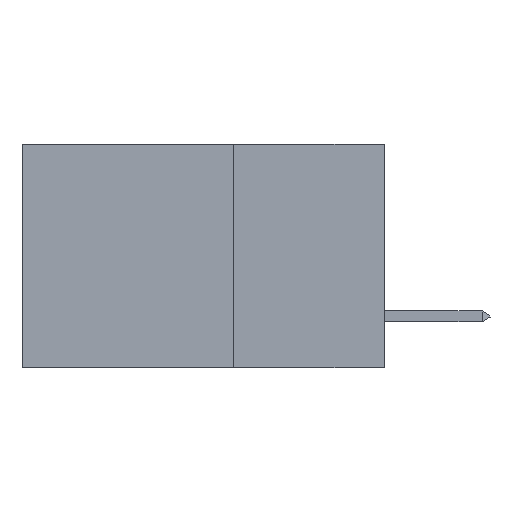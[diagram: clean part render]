
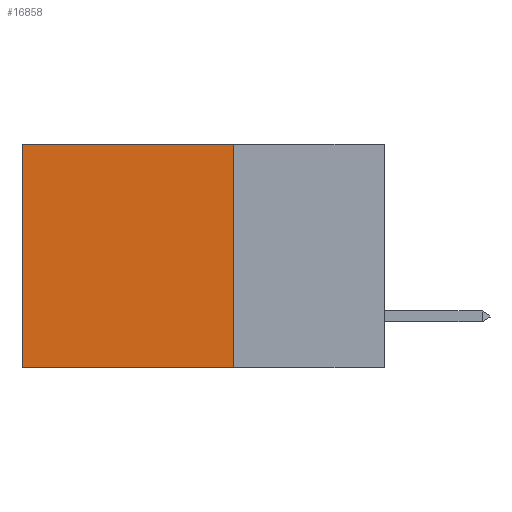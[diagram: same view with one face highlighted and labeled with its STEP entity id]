
A CAD part, left-side view. The second image highlights one B-rep face of the part: STEP entity #16858.
In plain terms, the highlighted planar face has unit normal (-1, 0, 0).
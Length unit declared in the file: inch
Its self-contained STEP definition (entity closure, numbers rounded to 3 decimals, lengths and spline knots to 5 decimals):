
#8 = DIRECTION ( 'NONE',  ( 0., 0., -1. ) ) ;
#34 = VERTEX_POINT ( 'NONE', #1742 ) ;
#244 = EDGE_LOOP ( 'NONE', ( #3949, #446, #4889, #4428 ) ) ;
#373 = CARTESIAN_POINT ( 'NONE',  ( 0.2875, 0.25, 0. ) ) ;
#446 = ORIENTED_EDGE ( 'NONE', *, *, #16270, .F. ) ;
#865 = VERTEX_POINT ( 'NONE', #12665 ) ;
#951 = EDGE_CURVE ( 'NONE', #34, #3635, #13948, .T. ) ;
#1742 = CARTESIAN_POINT ( 'NONE',  ( 0.2875, 0.6, 0. ) ) ;
#2558 = VERTEX_POINT ( 'NONE', #16355 ) ;
#2564 = CARTESIAN_POINT ( 'NONE',  ( 0.2875, 0.25, -0.37 ) ) ;
#3086 = CARTESIAN_POINT ( 'NONE',  ( 0.2875, 0.6, -0.37 ) ) ;
#3614 = FACE_OUTER_BOUND ( 'NONE', #244, .T. ) ;
#3635 = VERTEX_POINT ( 'NONE', #3086 ) ;
#3949 = ORIENTED_EDGE ( 'NONE', *, *, #951, .T. ) ;
#3950 = DIRECTION ( 'NONE',  ( 0., 1., 0. ) ) ;
#4428 = ORIENTED_EDGE ( 'NONE', *, *, #7048, .T. ) ;
#4889 = ORIENTED_EDGE ( 'NONE', *, *, #8742, .F. ) ;
#6504 = CARTESIAN_POINT ( 'NONE',  ( 0.2875, 0.25, 0. ) ) ;
#6998 = LINE ( 'NONE', #373, #10014 ) ;
#7048 = EDGE_CURVE ( 'NONE', #2558, #34, #6998, .T. ) ;
#7086 = DIRECTION ( 'NONE',  ( 0., 1., 0. ) ) ;
#7163 = VECTOR ( 'NONE', #8, 39.37008 ) ;
#7591 = VECTOR ( 'NONE', #12647, 39.37008 ) ;
#7809 = DIRECTION ( 'NONE',  ( 0., 0., -1. ) ) ;
#7985 = LINE ( 'NONE', #10564, #7163 ) ;
#8742 = EDGE_CURVE ( 'NONE', #2558, #865, #7985, .T. ) ;
#9997 = LINE ( 'NONE', #2564, #16313 ) ;
#10014 = VECTOR ( 'NONE', #7086, 39.37008 ) ;
#10540 = AXIS2_PLACEMENT_3D ( 'NONE', #6504, #15398, #7809 ) ;
#10564 = CARTESIAN_POINT ( 'NONE',  ( 0.2875, 0.25, 0. ) ) ;
#12647 = DIRECTION ( 'NONE',  ( 0., 0., -1. ) ) ;
#12665 = CARTESIAN_POINT ( 'NONE',  ( 0.2875, 0.25, -0.37 ) ) ;
#12973 = CARTESIAN_POINT ( 'NONE',  ( 0.2875, 0.6, 0. ) ) ;
#13948 = LINE ( 'NONE', #12973, #7591 ) ;
#15398 = DIRECTION ( 'NONE',  ( 1., 0., 0. ) ) ;
#16270 = EDGE_CURVE ( 'NONE', #865, #3635, #9997, .T. ) ;
#16313 = VECTOR ( 'NONE', #3950, 39.37008 ) ;
#16355 = CARTESIAN_POINT ( 'NONE',  ( 0.2875, 0.25, 0. ) ) ;
#16611 = PLANE ( 'NONE',  #10540 ) ;
#16858 = ADVANCED_FACE ( 'NONE', ( #3614 ), #16611, .F. ) ;
